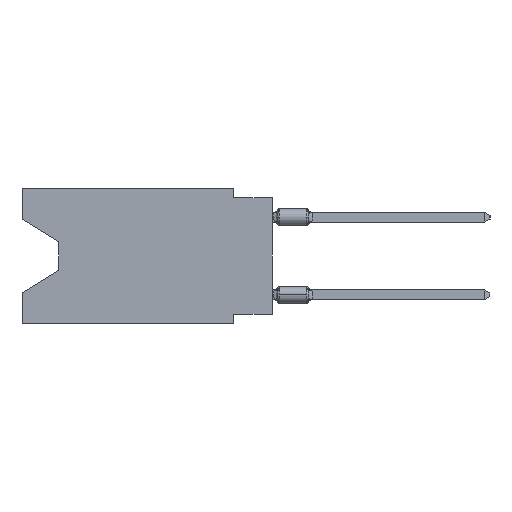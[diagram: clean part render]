
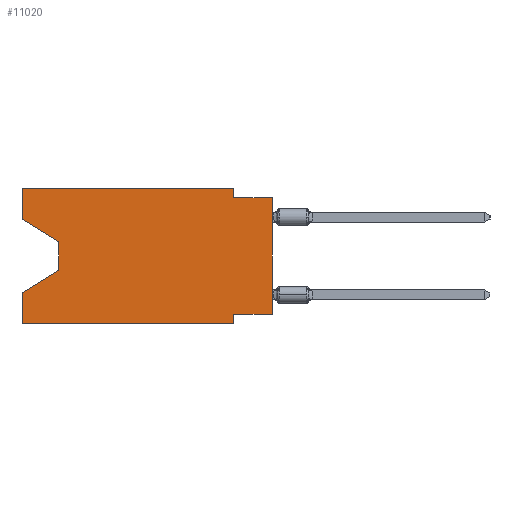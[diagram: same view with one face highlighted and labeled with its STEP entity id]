
A CAD part, left-side view. The second image highlights one B-rep face of the part: STEP entity #11020.
In plain terms, the highlighted planar face has unit normal (-1, 0, 0).
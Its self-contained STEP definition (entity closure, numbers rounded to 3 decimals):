
#121 = CARTESIAN_POINT ( 'NONE',  ( 0., 16.383, -2.038 ) ) ;
#526 = VECTOR ( 'NONE', #16613, 1000. ) ;
#605 = FACE_OUTER_BOUND ( 'NONE', #4183, .T. ) ;
#1720 = ORIENTED_EDGE ( 'NONE', *, *, #23055, .T. ) ;
#1763 = CARTESIAN_POINT ( 'NONE',  ( 0., 16.383, 0. ) ) ;
#2224 = LINE ( 'NONE', #16079, #17001 ) ;
#2818 = LINE ( 'NONE', #18188, #16264 ) ;
#3471 = ORIENTED_EDGE ( 'NONE', *, *, #13240, .F. ) ;
#3564 = VECTOR ( 'NONE', #8389, 1000. ) ;
#3759 = LINE ( 'NONE', #11394, #5218 ) ;
#3776 = DIRECTION ( 'NONE',  ( 0., -1., 0. ) ) ;
#3867 = DIRECTION ( 'NONE',  ( 0., -0.855, -0.519 ) ) ;
#4183 = EDGE_LOOP ( 'NONE', ( #20084, #6227, #18501, #11370, #1720, #11365, #14793, #17531, #23108, #22337, #14061, #3471 ) ) ;
#4195 = CARTESIAN_POINT ( 'NONE',  ( 0., 13.97, -5.385 ) ) ;
#4470 = CARTESIAN_POINT ( 'NONE',  ( 0., 2.54, 0. ) ) ;
#4673 = VECTOR ( 'NONE', #3867, 1000. ) ;
#4759 = LINE ( 'NONE', #22112, #8406 ) ;
#4877 = DIRECTION ( 'NONE',  ( 0., 0., -1. ) ) ;
#5218 = VECTOR ( 'NONE', #7645, 1000. ) ;
#5473 = DIRECTION ( 'NONE',  ( 0., -1., 0. ) ) ;
#5678 = VERTEX_POINT ( 'NONE', #23079 ) ;
#5987 = DIRECTION ( 'NONE',  ( 0., 1., 0. ) ) ;
#6129 = CARTESIAN_POINT ( 'NONE',  ( 0., 16.383, 0. ) ) ;
#6227 = ORIENTED_EDGE ( 'NONE', *, *, #9849, .T. ) ;
#6528 = LINE ( 'NONE', #22000, #3564 ) ;
#6631 = CARTESIAN_POINT ( 'NONE',  ( 0., 16.383, 0. ) ) ;
#6866 = EDGE_CURVE ( 'NONE', #16266, #19011, #2224, .T. ) ;
#7003 = LINE ( 'NONE', #6631, #526 ) ;
#7101 = VECTOR ( 'NONE', #23640, 1000. ) ;
#7484 = CARTESIAN_POINT ( 'NONE',  ( 0., 0., -8.255 ) ) ;
#7613 = CARTESIAN_POINT ( 'NONE',  ( 0., 13.97, -3.505 ) ) ;
#7645 = DIRECTION ( 'NONE',  ( 0., 0., -1. ) ) ;
#7886 = DIRECTION ( 'NONE',  ( 0., 0., 1. ) ) ;
#8035 = CARTESIAN_POINT ( 'NONE',  ( 0., 0., 0. ) ) ;
#8114 = VERTEX_POINT ( 'NONE', #21484 ) ;
#8124 = LINE ( 'NONE', #10003, #9163 ) ;
#8179 = EDGE_CURVE ( 'NONE', #8114, #19011, #8124, .T. ) ;
#8352 = DIRECTION ( 'NONE',  ( 0., 0., -1. ) ) ;
#8389 = DIRECTION ( 'NONE',  ( 0., -1., 0. ) ) ;
#8406 = VECTOR ( 'NONE', #4877, 1000. ) ;
#8521 = LINE ( 'NONE', #8035, #7101 ) ;
#9163 = VECTOR ( 'NONE', #7886, 1000. ) ;
#9606 = CARTESIAN_POINT ( 'NONE',  ( 0., 16.383, -6.852 ) ) ;
#9849 = EDGE_CURVE ( 'NONE', #20253, #16266, #2818, .T. ) ;
#9850 = DIRECTION ( 'NONE',  ( 0., 0.855, -0.519 ) ) ;
#10003 = CARTESIAN_POINT ( 'NONE',  ( 0., 16.383, 0. ) ) ;
#10452 = DIRECTION ( 'NONE',  ( 0., 0., -1. ) ) ;
#11020 = ADVANCED_FACE ( 'NONE', ( #605 ), #23219, .F. ) ;
#11069 = CARTESIAN_POINT ( 'NONE',  ( 0., 2.54, -0.635 ) ) ;
#11365 = ORIENTED_EDGE ( 'NONE', *, *, #19899, .F. ) ;
#11370 = ORIENTED_EDGE ( 'NONE', *, *, #8179, .F. ) ;
#11394 = CARTESIAN_POINT ( 'NONE',  ( 0., 2.54, -8.89 ) ) ;
#11540 = CARTESIAN_POINT ( 'NONE',  ( 0., 16.383, 0. ) ) ;
#12031 = CARTESIAN_POINT ( 'NONE',  ( 0., 0., -8.255 ) ) ;
#13240 = EDGE_CURVE ( 'NONE', #22196, #18701, #7003, .T. ) ;
#13995 = VERTEX_POINT ( 'NONE', #12031 ) ;
#14061 = ORIENTED_EDGE ( 'NONE', *, *, #18179, .F. ) ;
#14793 = ORIENTED_EDGE ( 'NONE', *, *, #19006, .F. ) ;
#14800 = VERTEX_POINT ( 'NONE', #4470 ) ;
#15450 = VERTEX_POINT ( 'NONE', #11069 ) ;
#15843 = EDGE_CURVE ( 'NONE', #22196, #20253, #21110, .T. ) ;
#16079 = CARTESIAN_POINT ( 'NONE',  ( 0., 13.97, -5.385 ) ) ;
#16264 = VECTOR ( 'NONE', #10452, 1000. ) ;
#16266 = VERTEX_POINT ( 'NONE', #4195 ) ;
#16512 = EDGE_CURVE ( 'NONE', #13995, #24362, #8521, .T. ) ;
#16613 = DIRECTION ( 'NONE',  ( 0., 0., 1. ) ) ;
#17001 = VECTOR ( 'NONE', #9850, 1000. ) ;
#17286 = LINE ( 'NONE', #11540, #18717 ) ;
#17531 = ORIENTED_EDGE ( 'NONE', *, *, #16512, .T. ) ;
#17859 = CARTESIAN_POINT ( 'NONE',  ( 0., 2.54, -8.255 ) ) ;
#18171 = CARTESIAN_POINT ( 'NONE',  ( 0., 0., -0.635 ) ) ;
#18179 = EDGE_CURVE ( 'NONE', #18701, #14800, #17286, .T. ) ;
#18188 = CARTESIAN_POINT ( 'NONE',  ( 0., 13.97, -3.505 ) ) ;
#18501 = ORIENTED_EDGE ( 'NONE', *, *, #6866, .T. ) ;
#18701 = VERTEX_POINT ( 'NONE', #1763 ) ;
#18717 = VECTOR ( 'NONE', #3776, 1000. ) ;
#18778 = VERTEX_POINT ( 'NONE', #17859 ) ;
#19006 = EDGE_CURVE ( 'NONE', #13995, #18778, #20851, .T. ) ;
#19011 = VERTEX_POINT ( 'NONE', #9606 ) ;
#19613 = DIRECTION ( 'NONE',  ( 1., 0., 0. ) ) ;
#19899 = EDGE_CURVE ( 'NONE', #18778, #5678, #3759, .T. ) ;
#20084 = ORIENTED_EDGE ( 'NONE', *, *, #15843, .T. ) ;
#20253 = VERTEX_POINT ( 'NONE', #7613 ) ;
#20478 = CARTESIAN_POINT ( 'NONE',  ( 0., 0., -0.635 ) ) ;
#20851 = LINE ( 'NONE', #7484, #21509 ) ;
#21110 = LINE ( 'NONE', #121, #4673 ) ;
#21484 = CARTESIAN_POINT ( 'NONE',  ( 0., 16.383, -8.89 ) ) ;
#21509 = VECTOR ( 'NONE', #5987, 1000. ) ;
#21770 = EDGE_CURVE ( 'NONE', #14800, #15450, #4759, .T. ) ;
#21991 = VECTOR ( 'NONE', #5473, 1000. ) ;
#22000 = CARTESIAN_POINT ( 'NONE',  ( 0., 16.383, -8.89 ) ) ;
#22112 = CARTESIAN_POINT ( 'NONE',  ( 0., 2.54, 0. ) ) ;
#22196 = VERTEX_POINT ( 'NONE', #23217 ) ;
#22332 = LINE ( 'NONE', #20478, #21991 ) ;
#22337 = ORIENTED_EDGE ( 'NONE', *, *, #21770, .F. ) ;
#22394 = EDGE_CURVE ( 'NONE', #15450, #24362, #22332, .T. ) ;
#23055 = EDGE_CURVE ( 'NONE', #8114, #5678, #6528, .T. ) ;
#23079 = CARTESIAN_POINT ( 'NONE',  ( 0., 2.54, -8.89 ) ) ;
#23108 = ORIENTED_EDGE ( 'NONE', *, *, #22394, .F. ) ;
#23217 = CARTESIAN_POINT ( 'NONE',  ( 0., 16.383, -2.038 ) ) ;
#23219 = PLANE ( 'NONE',  #23500 ) ;
#23500 = AXIS2_PLACEMENT_3D ( 'NONE', #6129, #19613, #8352 ) ;
#23640 = DIRECTION ( 'NONE',  ( 0., 0., 1. ) ) ;
#24362 = VERTEX_POINT ( 'NONE', #18171 ) ;
